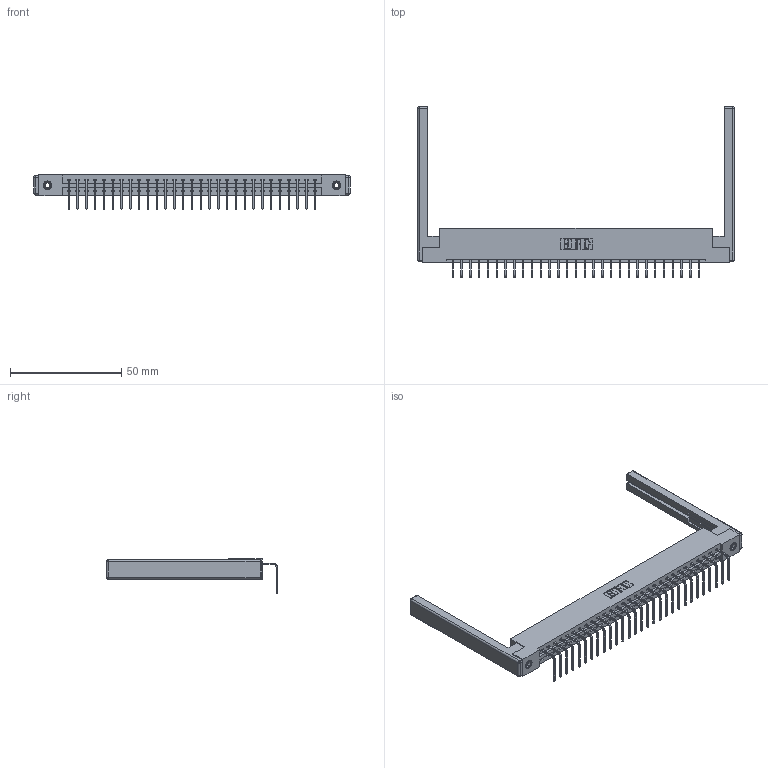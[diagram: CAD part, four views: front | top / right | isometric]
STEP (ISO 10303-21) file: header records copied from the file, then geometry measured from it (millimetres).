
FILE_DESCRIPTION (( 'STEP AP203' ), '1' );
FILE_NAME ('337-029-558-168.STEP', '2019-10-07T13:34:27', ( '' ), ( '' ), 'SwSTEP 2.0', 'SolidWorks 2016', '' );
FILE_SCHEMA (( 'CONFIG_CONTROL_DESIGN' ));
Length unit declared in the file: inch
Products named in the file (5): 307-220-068; 345-250-001_345-250-001-102; 345-292-001_558 Tail - 2; 337-029-558-168; 337 Part_Flush Mounting Lugs - 0.156 Dia-TI
Assembly tree (34 placements, depth 2):
  337-029-558-168
    337 Part_Flush Mounting Lugs - 0.156 Dia-TI
    345-292-001_558 Tail - 2  x29
    345-250-001_345-250-001-102  x2
    307-220-068  x2
Bounding box: 142.34 x 76.9 x 15.37 mm (x, y, z)
Volume: 19119.2 mm3; surface area: 19833.3 mm2
Topology: 34 solids, 34 shells, 2124 faces, 6327 edges, 4158 vertices
Faces by surface type: plane 1550, cylinder 550, cone 12, sphere 8, torus 4
Entity records: 26082 total; most frequent: CARTESIAN_POINT 4498, ORIENTED_EDGE 4452, DIRECTION 3886, EDGE_CURVE 2226, VECTOR 2048, LINE 2048, VERTEX_POINT 1474, AXIS2_PLACEMENT_3D 919
